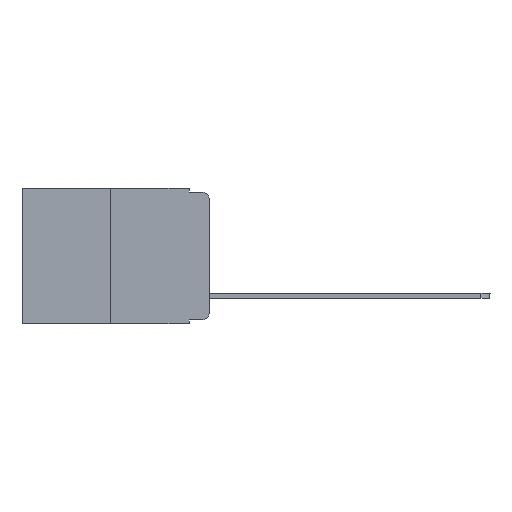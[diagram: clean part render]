
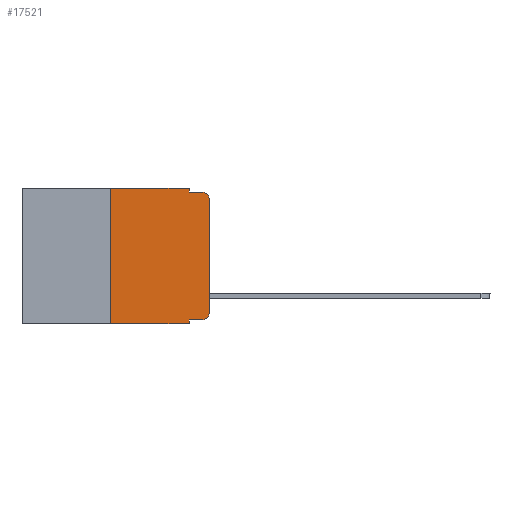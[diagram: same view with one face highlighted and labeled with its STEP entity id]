
A CAD part, left-side view. The second image highlights one B-rep face of the part: STEP entity #17521.
In plain terms, the highlighted planar face has unit normal (-1, 0, 0).
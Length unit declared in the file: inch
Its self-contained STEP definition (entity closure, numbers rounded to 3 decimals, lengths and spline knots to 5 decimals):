
#273 = DIRECTION ( 'NONE',  ( 0., 0., 1. ) ) ;
#653 = EDGE_CURVE ( 'NONE', #4864, #8420, #19896, .T. ) ;
#713 = AXIS2_PLACEMENT_3D ( 'NONE', #15494, #3580, #17183 ) ;
#1289 = VERTEX_POINT ( 'NONE', #6866 ) ;
#1589 = CARTESIAN_POINT ( 'NONE',  ( 0., 0.051, 0. ) ) ;
#1657 = ORIENTED_EDGE ( 'NONE', *, *, #6670, .T. ) ;
#1759 = CARTESIAN_POINT ( 'NONE',  ( 0., 0.473, 0. ) ) ;
#1898 = EDGE_CURVE ( 'NONE', #5864, #7935, #19785, .T. ) ;
#2384 = AXIS2_PLACEMENT_3D ( 'NONE', #17614, #7178, #12269 ) ;
#2452 = DIRECTION ( 'NONE',  ( 0., 0., -1. ) ) ;
#2839 = CIRCLE ( 'NONE', #713, 0.02 ) ;
#3098 = VECTOR ( 'NONE', #16080, 39.37008 ) ;
#3336 = LINE ( 'NONE', #5364, #3558 ) ;
#3389 = LINE ( 'NONE', #13987, #5881 ) ;
#3558 = VECTOR ( 'NONE', #10361, 39.37008 ) ;
#3580 = DIRECTION ( 'NONE',  ( -1., 0., 0. ) ) ;
#4410 = CARTESIAN_POINT ( 'NONE',  ( 0., 0.051, -0.333 ) ) ;
#4794 = CARTESIAN_POINT ( 'NONE',  ( 0., 0.051, -0.01 ) ) ;
#4864 = VERTEX_POINT ( 'NONE', #13494 ) ;
#5364 = CARTESIAN_POINT ( 'NONE',  ( 0., 0.051, -0.01 ) ) ;
#5819 = VERTEX_POINT ( 'NONE', #13669 ) ;
#5864 = VERTEX_POINT ( 'NONE', #12015 ) ;
#5881 = VECTOR ( 'NONE', #273, 39.37008 ) ;
#5939 = CARTESIAN_POINT ( 'NONE',  ( 0., 0.051, -0.333 ) ) ;
#5947 = EDGE_LOOP ( 'NONE', ( #1657, #17089, #16458, #6110, #20675, #18134, #20115, #8834, #14390, #20456 ) ) ;
#6034 = LINE ( 'NONE', #7629, #15490 ) ;
#6110 = ORIENTED_EDGE ( 'NONE', *, *, #14471, .F. ) ;
#6294 = LINE ( 'NONE', #15059, #21920 ) ;
#6670 = EDGE_CURVE ( 'NONE', #1289, #5864, #6034, .T. ) ;
#6866 = CARTESIAN_POINT ( 'NONE',  ( 0., 0., -0.313 ) ) ;
#7154 = VERTEX_POINT ( 'NONE', #20825 ) ;
#7178 = DIRECTION ( 'NONE',  ( -1., 0., 0. ) ) ;
#7629 = CARTESIAN_POINT ( 'NONE',  ( 0., 0., 0. ) ) ;
#7825 = EDGE_CURVE ( 'NONE', #4864, #5819, #3389, .T. ) ;
#7925 = LINE ( 'NONE', #17704, #13126 ) ;
#7935 = VERTEX_POINT ( 'NONE', #12730 ) ;
#8198 = VECTOR ( 'NONE', #9177, 39.37008 ) ;
#8420 = VERTEX_POINT ( 'NONE', #19198 ) ;
#8580 = DIRECTION ( 'NONE',  ( 0., 0., -1. ) ) ;
#8834 = ORIENTED_EDGE ( 'NONE', *, *, #12093, .F. ) ;
#9177 = DIRECTION ( 'NONE',  ( 0., -1., 0. ) ) ;
#9415 = EDGE_CURVE ( 'NONE', #5819, #14940, #6294, .T. ) ;
#9557 = DIRECTION ( 'NONE',  ( 0., -1., 0. ) ) ;
#9999 = DIRECTION ( 'NONE',  ( 1., 0., 0. ) ) ;
#10361 = DIRECTION ( 'NONE',  ( 0., -1., 0. ) ) ;
#11071 = CARTESIAN_POINT ( 'NONE',  ( 0., 0.051, 0. ) ) ;
#11156 = LINE ( 'NONE', #5939, #8198 ) ;
#11647 = VERTEX_POINT ( 'NONE', #4410 ) ;
#12015 = CARTESIAN_POINT ( 'NONE',  ( 0., 0., -0.03 ) ) ;
#12093 = EDGE_CURVE ( 'NONE', #11647, #8420, #14517, .T. ) ;
#12269 = DIRECTION ( 'NONE',  ( 0., 0., -1. ) ) ;
#12730 = CARTESIAN_POINT ( 'NONE',  ( 0., 0.02, -0.01 ) ) ;
#13126 = VECTOR ( 'NONE', #2452, 39.37008 ) ;
#13316 = PLANE ( 'NONE',  #18911 ) ;
#13363 = VECTOR ( 'NONE', #9557, 39.37008 ) ;
#13494 = CARTESIAN_POINT ( 'NONE',  ( 0., 0.25, -0.343 ) ) ;
#13669 = CARTESIAN_POINT ( 'NONE',  ( 0., 0.25, 0. ) ) ;
#13987 = CARTESIAN_POINT ( 'NONE',  ( 0., 0.25, 0. ) ) ;
#14101 = VERTEX_POINT ( 'NONE', #4794 ) ;
#14390 = ORIENTED_EDGE ( 'NONE', *, *, #20961, .T. ) ;
#14471 = EDGE_CURVE ( 'NONE', #14940, #14101, #7925, .T. ) ;
#14517 = LINE ( 'NONE', #11071, #3098 ) ;
#14671 = CARTESIAN_POINT ( 'NONE',  ( 0., 0.473, -0.343 ) ) ;
#14940 = VERTEX_POINT ( 'NONE', #1589 ) ;
#15059 = CARTESIAN_POINT ( 'NONE',  ( 0., 0.473, 0. ) ) ;
#15490 = VECTOR ( 'NONE', #19175, 39.37008 ) ;
#15494 = CARTESIAN_POINT ( 'NONE',  ( 0., 0.02, -0.313 ) ) ;
#16080 = DIRECTION ( 'NONE',  ( 0., 0., -1. ) ) ;
#16458 = ORIENTED_EDGE ( 'NONE', *, *, #21265, .F. ) ;
#17089 = ORIENTED_EDGE ( 'NONE', *, *, #1898, .T. ) ;
#17183 = DIRECTION ( 'NONE',  ( 0., 0., -1. ) ) ;
#17521 = ADVANCED_FACE ( 'NONE', ( #20472 ), #13316, .F. ) ;
#17614 = CARTESIAN_POINT ( 'NONE',  ( 0., 0.02, -0.03 ) ) ;
#17704 = CARTESIAN_POINT ( 'NONE',  ( 0., 0.051, 0. ) ) ;
#18134 = ORIENTED_EDGE ( 'NONE', *, *, #7825, .F. ) ;
#18911 = AXIS2_PLACEMENT_3D ( 'NONE', #1759, #9999, #8580 ) ;
#19175 = DIRECTION ( 'NONE',  ( 0., 0., 1. ) ) ;
#19198 = CARTESIAN_POINT ( 'NONE',  ( 0., 0.051, -0.343 ) ) ;
#19785 = CIRCLE ( 'NONE', #2384, 0.02 ) ;
#19896 = LINE ( 'NONE', #14671, #13363 ) ;
#20115 = ORIENTED_EDGE ( 'NONE', *, *, #653, .T. ) ;
#20456 = ORIENTED_EDGE ( 'NONE', *, *, #20848, .T. ) ;
#20472 = FACE_OUTER_BOUND ( 'NONE', #5947, .T. ) ;
#20675 = ORIENTED_EDGE ( 'NONE', *, *, #9415, .F. ) ;
#20825 = CARTESIAN_POINT ( 'NONE',  ( 0., 0.02, -0.333 ) ) ;
#20848 = EDGE_CURVE ( 'NONE', #7154, #1289, #2839, .T. ) ;
#20961 = EDGE_CURVE ( 'NONE', #11647, #7154, #11156, .T. ) ;
#21265 = EDGE_CURVE ( 'NONE', #14101, #7935, #3336, .T. ) ;
#21874 = DIRECTION ( 'NONE',  ( 0., -1., 0. ) ) ;
#21920 = VECTOR ( 'NONE', #21874, 39.37008 ) ;
